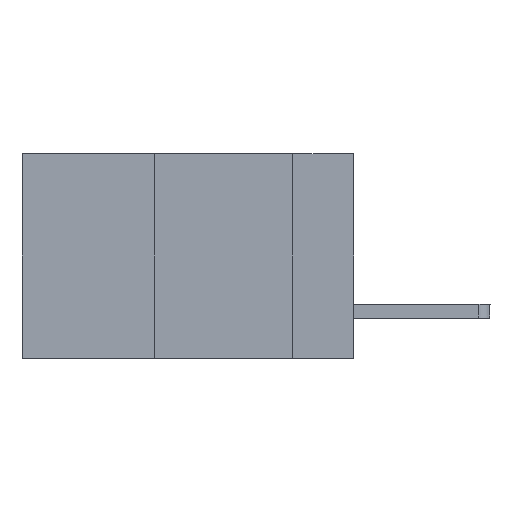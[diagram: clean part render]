
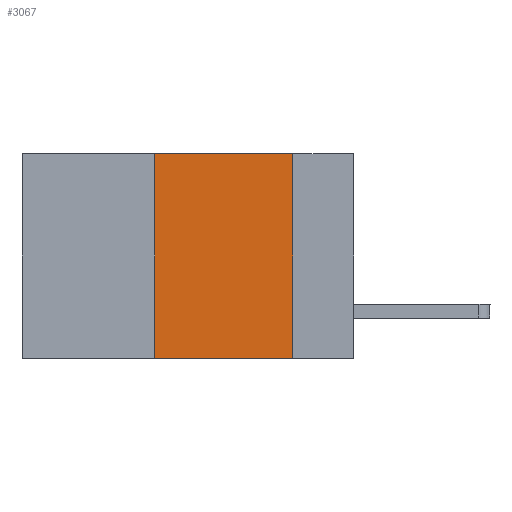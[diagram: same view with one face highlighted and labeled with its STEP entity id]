
A CAD part, left-side view. The second image highlights one B-rep face of the part: STEP entity #3067.
In plain terms, the highlighted planar face has unit normal (-1, 0, 0).
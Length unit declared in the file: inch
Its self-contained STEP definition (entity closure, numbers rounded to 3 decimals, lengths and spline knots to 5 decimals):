
#586 = CARTESIAN_POINT ( 'NONE',  ( 0., 0.6, -0.37 ) ) ;
#800 = CARTESIAN_POINT ( 'NONE',  ( 0., 0.36, -0.37 ) ) ;
#1420 = FACE_OUTER_BOUND ( 'NONE', #9160, .T. ) ;
#1464 = VERTEX_POINT ( 'NONE', #1917 ) ;
#1473 = VECTOR ( 'NONE', #2401, 39.37008 ) ;
#1748 = EDGE_CURVE ( 'NONE', #4331, #4729, #8547, .T. ) ;
#1836 = CARTESIAN_POINT ( 'NONE',  ( 0., 0.11, 0. ) ) ;
#1917 = CARTESIAN_POINT ( 'NONE',  ( 0., 0.36, 0. ) ) ;
#2401 = DIRECTION ( 'NONE',  ( 0., 0., -1. ) ) ;
#2430 = VERTEX_POINT ( 'NONE', #1836 ) ;
#2597 = PLANE ( 'NONE',  #8770 ) ;
#2945 = ORIENTED_EDGE ( 'NONE', *, *, #4643, .F. ) ;
#3067 = ADVANCED_FACE ( 'NONE', ( #1420 ), #2597, .F. ) ;
#3189 = LINE ( 'NONE', #8203, #5904 ) ;
#3308 = ORIENTED_EDGE ( 'NONE', *, *, #6115, .F. ) ;
#3354 = CARTESIAN_POINT ( 'NONE',  ( 0., 0.6, 0. ) ) ;
#3990 = DIRECTION ( 'NONE',  ( 0., -1., 0. ) ) ;
#4243 = DIRECTION ( 'NONE',  ( 1., 0., 0. ) ) ;
#4263 = ORIENTED_EDGE ( 'NONE', *, *, #7560, .F. ) ;
#4331 = VERTEX_POINT ( 'NONE', #800 ) ;
#4643 = EDGE_CURVE ( 'NONE', #4331, #1464, #3189, .T. ) ;
#4729 = VERTEX_POINT ( 'NONE', #5038 ) ;
#4853 = CARTESIAN_POINT ( 'NONE',  ( 0., 0.11, 0. ) ) ;
#5038 = CARTESIAN_POINT ( 'NONE',  ( 0., 0.11, -0.37 ) ) ;
#5904 = VECTOR ( 'NONE', #6688, 39.37008 ) ;
#6115 = EDGE_CURVE ( 'NONE', #2430, #4729, #9363, .T. ) ;
#6349 = DIRECTION ( 'NONE',  ( 0., -1., 0. ) ) ;
#6504 = LINE ( 'NONE', #8994, #7911 ) ;
#6688 = DIRECTION ( 'NONE',  ( 0., 0., 1. ) ) ;
#7096 = ORIENTED_EDGE ( 'NONE', *, *, #1748, .T. ) ;
#7560 = EDGE_CURVE ( 'NONE', #1464, #2430, #6504, .T. ) ;
#7911 = VECTOR ( 'NONE', #3990, 39.37008 ) ;
#8203 = CARTESIAN_POINT ( 'NONE',  ( 0., 0.36, 0. ) ) ;
#8435 = VECTOR ( 'NONE', #6349, 39.37008 ) ;
#8547 = LINE ( 'NONE', #586, #8435 ) ;
#8770 = AXIS2_PLACEMENT_3D ( 'NONE', #3354, #4243, #10058 ) ;
#8994 = CARTESIAN_POINT ( 'NONE',  ( 0., 0.6, 0. ) ) ;
#9160 = EDGE_LOOP ( 'NONE', ( #3308, #4263, #2945, #7096 ) ) ;
#9363 = LINE ( 'NONE', #4853, #1473 ) ;
#10058 = DIRECTION ( 'NONE',  ( 0., 0., -1. ) ) ;
